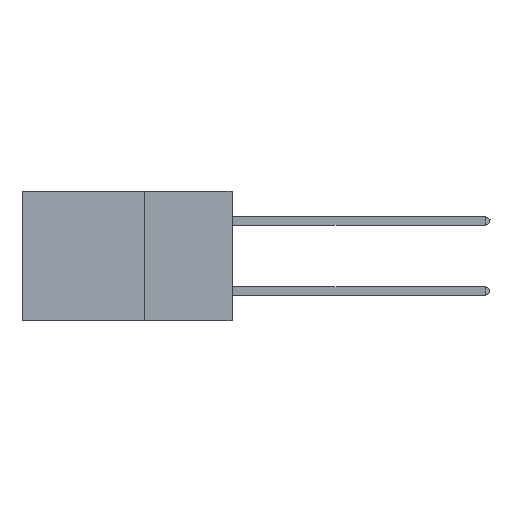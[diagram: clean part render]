
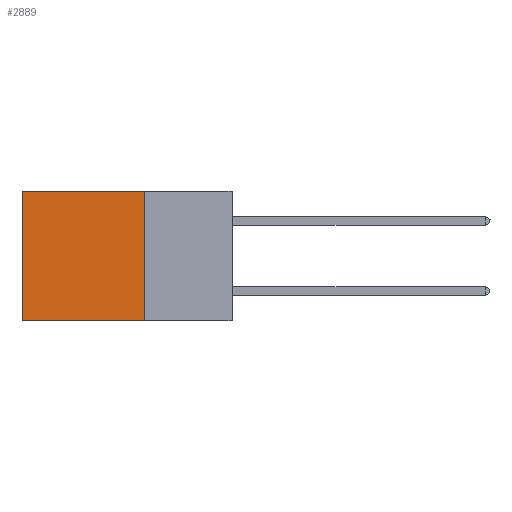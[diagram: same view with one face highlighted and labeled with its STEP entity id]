
A CAD part, left-side view. The second image highlights one B-rep face of the part: STEP entity #2889.
In plain terms, the highlighted planar face has unit normal (-1, 0, 0).
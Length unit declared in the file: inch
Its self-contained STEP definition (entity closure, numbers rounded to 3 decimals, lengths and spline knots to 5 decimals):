
#199 = EDGE_CURVE ( 'NONE', #2989, #10310, #16744, .T. ) ;
#907 = ORIENTED_EDGE ( 'NONE', *, *, #19200, .F. ) ;
#1150 = LINE ( 'NONE', #10454, #12149 ) ;
#1844 = CARTESIAN_POINT ( 'NONE',  ( 0.2875, 0.25, -0.37 ) ) ;
#1935 = VERTEX_POINT ( 'NONE', #12139 ) ;
#2748 = DIRECTION ( 'NONE',  ( 0., 0., -1. ) ) ;
#2889 = ADVANCED_FACE ( 'NONE', ( #16691 ), #19864, .F. ) ;
#2989 = VERTEX_POINT ( 'NONE', #8617 ) ;
#4095 = LINE ( 'NONE', #11964, #6089 ) ;
#5521 = VERTEX_POINT ( 'NONE', #13740 ) ;
#5859 = DIRECTION ( 'NONE',  ( 1., 0., 0. ) ) ;
#5955 = DIRECTION ( 'NONE',  ( 0., 0., -1. ) ) ;
#6089 = VECTOR ( 'NONE', #7457, 39.37008 ) ;
#6208 = CARTESIAN_POINT ( 'NONE',  ( 0.2875, 0.25, -0.37 ) ) ;
#6322 = EDGE_CURVE ( 'NONE', #2989, #1935, #4095, .T. ) ;
#7205 = VECTOR ( 'NONE', #2748, 39.37008 ) ;
#7398 = DIRECTION ( 'NONE',  ( 0., 0., -1. ) ) ;
#7457 = DIRECTION ( 'NONE',  ( 0., 1., 0. ) ) ;
#8617 = CARTESIAN_POINT ( 'NONE',  ( 0.2875, 0.25, 0. ) ) ;
#8869 = VECTOR ( 'NONE', #17477, 39.37008 ) ;
#9522 = LINE ( 'NONE', #1844, #8869 ) ;
#10310 = VERTEX_POINT ( 'NONE', #6208 ) ;
#10454 = CARTESIAN_POINT ( 'NONE',  ( 0.2875, 0.6, 0. ) ) ;
#11964 = CARTESIAN_POINT ( 'NONE',  ( 0.2875, 0.25, 0. ) ) ;
#12139 = CARTESIAN_POINT ( 'NONE',  ( 0.2875, 0.6, 0. ) ) ;
#12149 = VECTOR ( 'NONE', #5955, 39.37008 ) ;
#13394 = ORIENTED_EDGE ( 'NONE', *, *, #199, .F. ) ;
#13740 = CARTESIAN_POINT ( 'NONE',  ( 0.2875, 0.6, -0.37 ) ) ;
#13988 = EDGE_LOOP ( 'NONE', ( #19630, #907, #13394, #18344 ) ) ;
#14964 = AXIS2_PLACEMENT_3D ( 'NONE', #16792, #5859, #7398 ) ;
#15225 = CARTESIAN_POINT ( 'NONE',  ( 0.2875, 0.25, 0. ) ) ;
#16691 = FACE_OUTER_BOUND ( 'NONE', #13988, .T. ) ;
#16744 = LINE ( 'NONE', #15225, #7205 ) ;
#16792 = CARTESIAN_POINT ( 'NONE',  ( 0.2875, 0.25, 0. ) ) ;
#17477 = DIRECTION ( 'NONE',  ( 0., 1., 0. ) ) ;
#18344 = ORIENTED_EDGE ( 'NONE', *, *, #6322, .T. ) ;
#19200 = EDGE_CURVE ( 'NONE', #10310, #5521, #9522, .T. ) ;
#19630 = ORIENTED_EDGE ( 'NONE', *, *, #19678, .T. ) ;
#19678 = EDGE_CURVE ( 'NONE', #1935, #5521, #1150, .T. ) ;
#19864 = PLANE ( 'NONE',  #14964 ) ;
